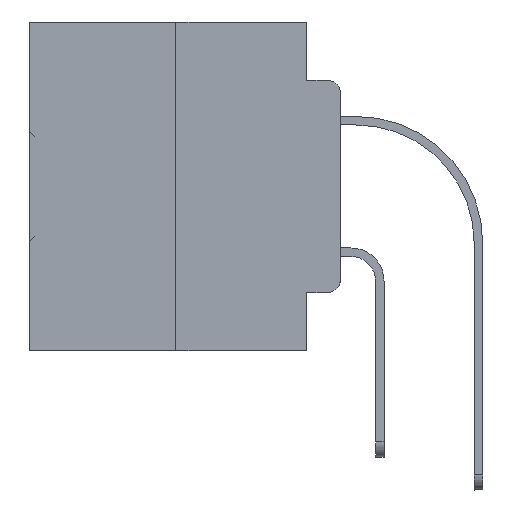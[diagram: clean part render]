
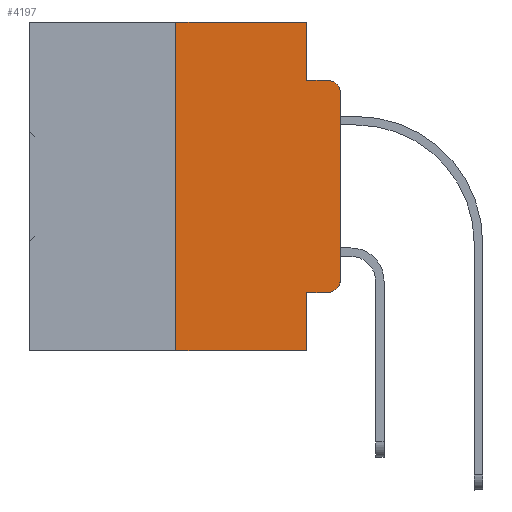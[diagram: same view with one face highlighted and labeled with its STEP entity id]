
A CAD part, left-side view. The second image highlights one B-rep face of the part: STEP entity #4197.
In plain terms, the highlighted planar face has unit normal (-1, 0, 0).
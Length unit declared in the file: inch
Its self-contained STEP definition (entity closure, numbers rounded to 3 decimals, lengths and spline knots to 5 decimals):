
#551 = VERTEX_POINT ( 'NONE', #31970 ) ;
#659 = VERTEX_POINT ( 'NONE', #32353 ) ;
#662 = CARTESIAN_POINT ( 'NONE',  ( 0., 0.02, -0.3915 ) ) ;
#698 = CIRCLE ( 'NONE', #12275, 0.02 ) ;
#1325 = DIRECTION ( 'NONE',  ( -1., 0., 0. ) ) ;
#2196 = EDGE_CURVE ( 'NONE', #35020, #30128, #16172, .T. ) ;
#2248 = VERTEX_POINT ( 'NONE', #30877 ) ;
#2249 = DIRECTION ( 'NONE',  ( 0., 0., -1. ) ) ;
#2524 = ORIENTED_EDGE ( 'NONE', *, *, #2196, .F. ) ;
#3357 = CARTESIAN_POINT ( 'NONE',  ( 0., 0.051, 0. ) ) ;
#4197 = ADVANCED_FACE ( 'NONE', ( #12852 ), #21220, .F. ) ;
#4365 = CARTESIAN_POINT ( 'NONE',  ( 0., 0.02, -0.4115 ) ) ;
#4413 = LINE ( 'NONE', #7252, #35281 ) ;
#5353 = VECTOR ( 'NONE', #7594, 39.37008 ) ;
#5739 = CARTESIAN_POINT ( 'NONE',  ( 0., 0.051, -0.4115 ) ) ;
#5972 = CARTESIAN_POINT ( 'NONE',  ( 0., 0., 0. ) ) ;
#6256 = CARTESIAN_POINT ( 'NONE',  ( 0., 0.051, -0.5 ) ) ;
#6646 = CARTESIAN_POINT ( 'NONE',  ( 0., 0.02, -0.1085 ) ) ;
#7252 = CARTESIAN_POINT ( 'NONE',  ( 0., 0.473, -0.5 ) ) ;
#7324 = ORIENTED_EDGE ( 'NONE', *, *, #18651, .T. ) ;
#7594 = DIRECTION ( 'NONE',  ( 0., -1., 0. ) ) ;
#7769 = CARTESIAN_POINT ( 'NONE',  ( 0., 0.051, -0.0885 ) ) ;
#9696 = ORIENTED_EDGE ( 'NONE', *, *, #35350, .F. ) ;
#10210 = EDGE_CURVE ( 'NONE', #23457, #10631, #36487, .T. ) ;
#10631 = VERTEX_POINT ( 'NONE', #20445 ) ;
#11717 = LINE ( 'NONE', #5972, #36720 ) ;
#12275 = AXIS2_PLACEMENT_3D ( 'NONE', #6646, #1325, #27451 ) ;
#12852 = FACE_OUTER_BOUND ( 'NONE', #17252, .T. ) ;
#13146 = LINE ( 'NONE', #21713, #36011 ) ;
#13536 = AXIS2_PLACEMENT_3D ( 'NONE', #27161, #21045, #33281 ) ;
#13623 = CARTESIAN_POINT ( 'NONE',  ( 0., 0.051, 0. ) ) ;
#13870 = ORIENTED_EDGE ( 'NONE', *, *, #16461, .T. ) ;
#14104 = VECTOR ( 'NONE', #14890, 39.37008 ) ;
#14587 = CARTESIAN_POINT ( 'NONE',  ( 0., 0.051, -0.0885 ) ) ;
#14890 = DIRECTION ( 'NONE',  ( 0., -1., 0. ) ) ;
#15634 = EDGE_CURVE ( 'NONE', #20866, #23457, #29192, .T. ) ;
#16053 = ORIENTED_EDGE ( 'NONE', *, *, #24528, .T. ) ;
#16172 = LINE ( 'NONE', #28382, #25090 ) ;
#16284 = LINE ( 'NONE', #13623, #21504 ) ;
#16461 = EDGE_CURVE ( 'NONE', #10631, #2248, #11717, .T. ) ;
#17252 = EDGE_LOOP ( 'NONE', ( #13870, #16053, #25389, #2524, #24654, #23342, #7324, #9696, #17466, #32783 ) ) ;
#17466 = ORIENTED_EDGE ( 'NONE', *, *, #15634, .T. ) ;
#17685 = EDGE_CURVE ( 'NONE', #30128, #659, #34129, .T. ) ;
#18514 = DIRECTION ( 'NONE',  ( 0., -1., 0. ) ) ;
#18651 = EDGE_CURVE ( 'NONE', #551, #28526, #4413, .T. ) ;
#19825 = EDGE_CURVE ( 'NONE', #35260, #35020, #21008, .T. ) ;
#19994 = AXIS2_PLACEMENT_3D ( 'NONE', #662, #29288, #37695 ) ;
#20445 = CARTESIAN_POINT ( 'NONE',  ( 0., 0., -0.3915 ) ) ;
#20649 = DIRECTION ( 'NONE',  ( 0., 0., 1. ) ) ;
#20866 = VERTEX_POINT ( 'NONE', #35457 ) ;
#21008 = LINE ( 'NONE', #34986, #34064 ) ;
#21045 = DIRECTION ( 'NONE',  ( 1., 0., 0. ) ) ;
#21220 = PLANE ( 'NONE',  #13536 ) ;
#21504 = VECTOR ( 'NONE', #36914, 39.37008 ) ;
#21713 = CARTESIAN_POINT ( 'NONE',  ( 0., 0.25, 0. ) ) ;
#21827 = EDGE_CURVE ( 'NONE', #551, #35260, #13146, .T. ) ;
#23342 = ORIENTED_EDGE ( 'NONE', *, *, #21827, .F. ) ;
#23457 = VERTEX_POINT ( 'NONE', #4365 ) ;
#24296 = CARTESIAN_POINT ( 'NONE',  ( 0., 0.25, 0. ) ) ;
#24528 = EDGE_CURVE ( 'NONE', #2248, #659, #698, .T. ) ;
#24654 = ORIENTED_EDGE ( 'NONE', *, *, #19825, .F. ) ;
#25090 = VECTOR ( 'NONE', #2249, 39.37008 ) ;
#25389 = ORIENTED_EDGE ( 'NONE', *, *, #17685, .F. ) ;
#27161 = CARTESIAN_POINT ( 'NONE',  ( 0., 0.473, 0. ) ) ;
#27451 = DIRECTION ( 'NONE',  ( 0., 0., -1. ) ) ;
#28382 = CARTESIAN_POINT ( 'NONE',  ( 0., 0.051, 0. ) ) ;
#28526 = VERTEX_POINT ( 'NONE', #6256 ) ;
#29192 = LINE ( 'NONE', #5739, #14104 ) ;
#29288 = DIRECTION ( 'NONE',  ( -1., 0., 0. ) ) ;
#30128 = VERTEX_POINT ( 'NONE', #14587 ) ;
#30877 = CARTESIAN_POINT ( 'NONE',  ( 0., 0., -0.1085 ) ) ;
#31970 = CARTESIAN_POINT ( 'NONE',  ( 0., 0.25, -0.5 ) ) ;
#32104 = DIRECTION ( 'NONE',  ( 0., -1., 0. ) ) ;
#32353 = CARTESIAN_POINT ( 'NONE',  ( 0., 0.02, -0.0885 ) ) ;
#32783 = ORIENTED_EDGE ( 'NONE', *, *, #10210, .T. ) ;
#33025 = DIRECTION ( 'NONE',  ( 0., 0., 1. ) ) ;
#33281 = DIRECTION ( 'NONE',  ( 0., 0., -1. ) ) ;
#34064 = VECTOR ( 'NONE', #32104, 39.37008 ) ;
#34129 = LINE ( 'NONE', #7769, #5353 ) ;
#34986 = CARTESIAN_POINT ( 'NONE',  ( 0., 0.473, 0. ) ) ;
#35020 = VERTEX_POINT ( 'NONE', #3357 ) ;
#35260 = VERTEX_POINT ( 'NONE', #24296 ) ;
#35281 = VECTOR ( 'NONE', #18514, 39.37008 ) ;
#35350 = EDGE_CURVE ( 'NONE', #20866, #28526, #16284, .T. ) ;
#35457 = CARTESIAN_POINT ( 'NONE',  ( 0., 0.051, -0.4115 ) ) ;
#36011 = VECTOR ( 'NONE', #33025, 39.37008 ) ;
#36487 = CIRCLE ( 'NONE', #19994, 0.02 ) ;
#36720 = VECTOR ( 'NONE', #20649, 39.37008 ) ;
#36914 = DIRECTION ( 'NONE',  ( 0., 0., -1. ) ) ;
#37695 = DIRECTION ( 'NONE',  ( 0., 0., -1. ) ) ;
